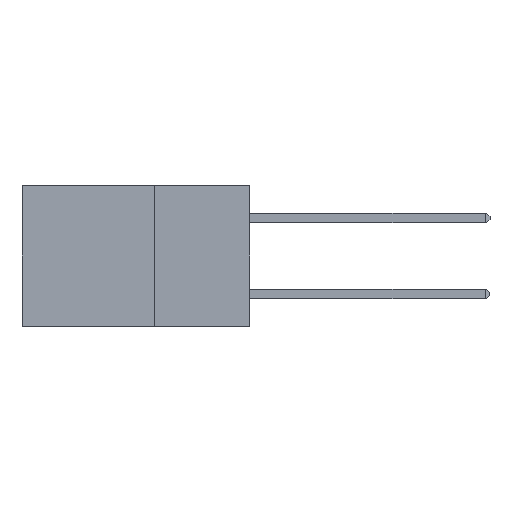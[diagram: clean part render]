
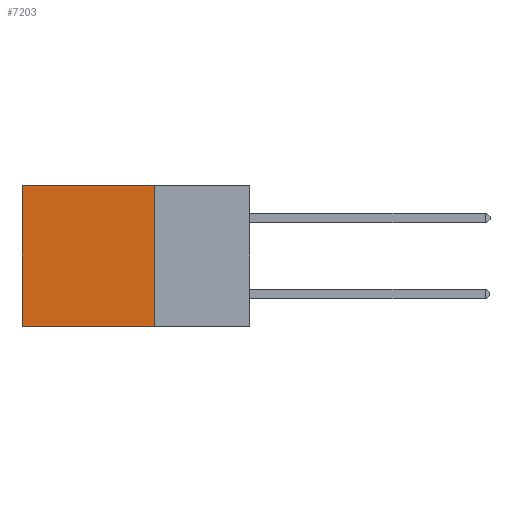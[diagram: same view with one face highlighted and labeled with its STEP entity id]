
A CAD part, left-side view. The second image highlights one B-rep face of the part: STEP entity #7203.
In plain terms, the highlighted planar face has unit normal (-1, 0, 0).
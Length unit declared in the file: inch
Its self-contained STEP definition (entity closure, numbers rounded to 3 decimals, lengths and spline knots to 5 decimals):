
#168 = CARTESIAN_POINT ( 'NONE',  ( 0.2875, 0.25, 0. ) ) ;
#309 = CARTESIAN_POINT ( 'NONE',  ( 0.2875, 0.25, -0.37 ) ) ;
#340 = CARTESIAN_POINT ( 'NONE',  ( 0.2875, 0.6, 0. ) ) ;
#594 = VECTOR ( 'NONE', #8931, 39.37008 ) ;
#1728 = CARTESIAN_POINT ( 'NONE',  ( 0.2875, 0.25, 0. ) ) ;
#2183 = LINE ( 'NONE', #340, #14949 ) ;
#2704 = CARTESIAN_POINT ( 'NONE',  ( 0.2875, 0.6, 0. ) ) ;
#2719 = VERTEX_POINT ( 'NONE', #2778 ) ;
#2778 = CARTESIAN_POINT ( 'NONE',  ( 0.2875, 0.25, 0. ) ) ;
#3282 = EDGE_CURVE ( 'NONE', #12095, #8843, #2183, .T. ) ;
#3630 = LINE ( 'NONE', #168, #594 ) ;
#4394 = LINE ( 'NONE', #1728, #13769 ) ;
#5708 = VERTEX_POINT ( 'NONE', #309 ) ;
#6451 = DIRECTION ( 'NONE',  ( 0., 0., -1. ) ) ;
#7203 = ADVANCED_FACE ( 'NONE', ( #11557 ), #13338, .F. ) ;
#7681 = ORIENTED_EDGE ( 'NONE', *, *, #11302, .F. ) ;
#7688 = LINE ( 'NONE', #12748, #10540 ) ;
#7917 = CARTESIAN_POINT ( 'NONE',  ( 0.2875, 0.6, -0.37 ) ) ;
#8472 = ORIENTED_EDGE ( 'NONE', *, *, #11631, .T. ) ;
#8697 = DIRECTION ( 'NONE',  ( 0., 0., -1. ) ) ;
#8843 = VERTEX_POINT ( 'NONE', #7917 ) ;
#8931 = DIRECTION ( 'NONE',  ( 0., 1., 0. ) ) ;
#9145 = ORIENTED_EDGE ( 'NONE', *, *, #3282, .T. ) ;
#9395 = AXIS2_PLACEMENT_3D ( 'NONE', #13371, #12636, #8697 ) ;
#10319 = ORIENTED_EDGE ( 'NONE', *, *, #12736, .F. ) ;
#10370 = DIRECTION ( 'NONE',  ( 0., 0., -1. ) ) ;
#10540 = VECTOR ( 'NONE', #15264, 39.37008 ) ;
#11302 = EDGE_CURVE ( 'NONE', #5708, #8843, #7688, .T. ) ;
#11557 = FACE_OUTER_BOUND ( 'NONE', #14509, .T. ) ;
#11631 = EDGE_CURVE ( 'NONE', #2719, #12095, #3630, .T. ) ;
#12095 = VERTEX_POINT ( 'NONE', #2704 ) ;
#12636 = DIRECTION ( 'NONE',  ( 1., 0., 0. ) ) ;
#12736 = EDGE_CURVE ( 'NONE', #2719, #5708, #4394, .T. ) ;
#12748 = CARTESIAN_POINT ( 'NONE',  ( 0.2875, 0.25, -0.37 ) ) ;
#13338 = PLANE ( 'NONE',  #9395 ) ;
#13371 = CARTESIAN_POINT ( 'NONE',  ( 0.2875, 0.25, 0. ) ) ;
#13769 = VECTOR ( 'NONE', #10370, 39.37008 ) ;
#14509 = EDGE_LOOP ( 'NONE', ( #9145, #7681, #10319, #8472 ) ) ;
#14949 = VECTOR ( 'NONE', #6451, 39.37008 ) ;
#15264 = DIRECTION ( 'NONE',  ( 0., 1., 0. ) ) ;
